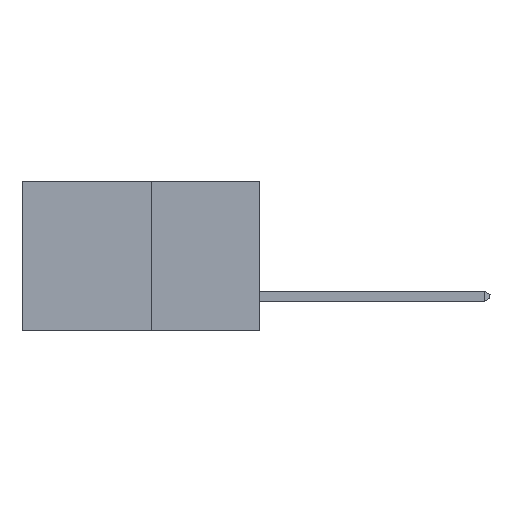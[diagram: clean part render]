
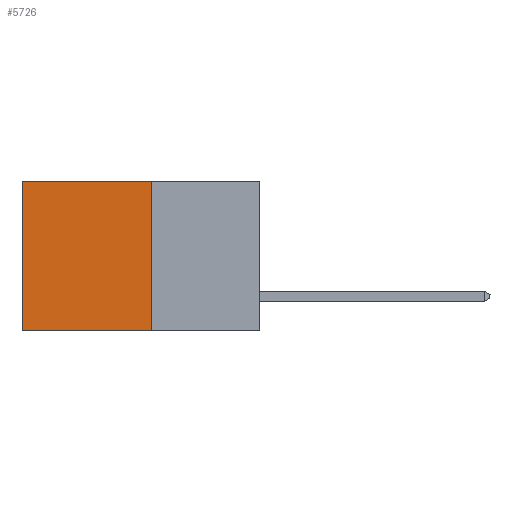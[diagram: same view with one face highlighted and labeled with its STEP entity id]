
A CAD part, left-side view. The second image highlights one B-rep face of the part: STEP entity #5726.
In plain terms, the highlighted planar face has unit normal (-1, 0, 0).
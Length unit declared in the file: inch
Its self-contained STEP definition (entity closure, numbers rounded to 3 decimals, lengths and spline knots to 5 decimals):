
#897 = EDGE_CURVE ( 'NONE', #5594, #12483, #1157, .T. ) ;
#1157 = LINE ( 'NONE', #15299, #13688 ) ;
#2098 = ORIENTED_EDGE ( 'NONE', *, *, #10442, .T. ) ;
#2903 = VECTOR ( 'NONE', #10070, 39.37008 ) ;
#3883 = EDGE_LOOP ( 'NONE', ( #13974, #18800, #9740, #2098 ) ) ;
#4661 = EDGE_CURVE ( 'NONE', #7397, #12977, #5473, .T. ) ;
#5473 = LINE ( 'NONE', #17815, #12993 ) ;
#5594 = VERTEX_POINT ( 'NONE', #7365 ) ;
#5726 = ADVANCED_FACE ( 'NONE', ( #17986 ), #12730, .F. ) ;
#7365 = CARTESIAN_POINT ( 'NONE',  ( 0.277, 0.59, 0. ) ) ;
#7397 = VERTEX_POINT ( 'NONE', #14972 ) ;
#7826 = DIRECTION ( 'NONE',  ( 0., 1., 0. ) ) ;
#7918 = CARTESIAN_POINT ( 'NONE',  ( 0.277, 0.27, 0. ) ) ;
#8512 = CARTESIAN_POINT ( 'NONE',  ( 0.277, 0.59, -0.37 ) ) ;
#9105 = DIRECTION ( 'NONE',  ( 0., 0., -1. ) ) ;
#9740 = ORIENTED_EDGE ( 'NONE', *, *, #4661, .F. ) ;
#10070 = DIRECTION ( 'NONE',  ( 0., 1., 0. ) ) ;
#10154 = CARTESIAN_POINT ( 'NONE',  ( 0.277, 0.27, -0.37 ) ) ;
#10199 = VECTOR ( 'NONE', #7826, 39.37008 ) ;
#10208 = EDGE_CURVE ( 'NONE', #12977, #12483, #15365, .T. ) ;
#10442 = EDGE_CURVE ( 'NONE', #7397, #5594, #18550, .T. ) ;
#11039 = CARTESIAN_POINT ( 'NONE',  ( 0.277, 0.27, -0.37 ) ) ;
#11870 = DIRECTION ( 'NONE',  ( 0., 0., -1. ) ) ;
#12483 = VERTEX_POINT ( 'NONE', #8512 ) ;
#12580 = DIRECTION ( 'NONE',  ( 1., 0., 0. ) ) ;
#12730 = PLANE ( 'NONE',  #19226 ) ;
#12837 = CARTESIAN_POINT ( 'NONE',  ( 0.277, 0.27, -0.37 ) ) ;
#12977 = VERTEX_POINT ( 'NONE', #11039 ) ;
#12993 = VECTOR ( 'NONE', #17520, 39.37008 ) ;
#13688 = VECTOR ( 'NONE', #9105, 39.37008 ) ;
#13974 = ORIENTED_EDGE ( 'NONE', *, *, #897, .T. ) ;
#14972 = CARTESIAN_POINT ( 'NONE',  ( 0.277, 0.27, 0. ) ) ;
#15299 = CARTESIAN_POINT ( 'NONE',  ( 0.277, 0.59, -0.37 ) ) ;
#15365 = LINE ( 'NONE', #10154, #2903 ) ;
#17520 = DIRECTION ( 'NONE',  ( 0., 0., -1. ) ) ;
#17815 = CARTESIAN_POINT ( 'NONE',  ( 0.277, 0.27, -0.37 ) ) ;
#17986 = FACE_OUTER_BOUND ( 'NONE', #3883, .T. ) ;
#18550 = LINE ( 'NONE', #7918, #10199 ) ;
#18800 = ORIENTED_EDGE ( 'NONE', *, *, #10208, .F. ) ;
#19226 = AXIS2_PLACEMENT_3D ( 'NONE', #12837, #12580, #11870 ) ;
